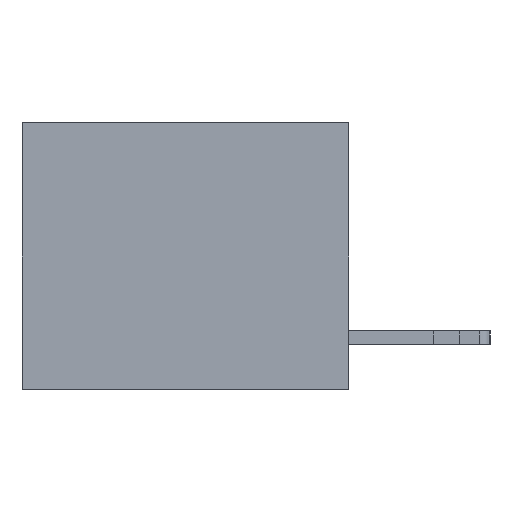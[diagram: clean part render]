
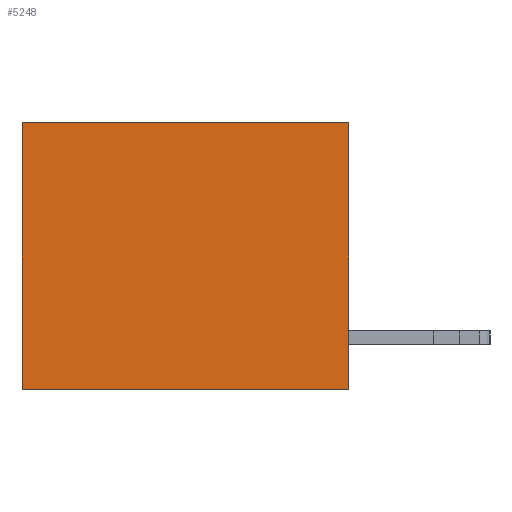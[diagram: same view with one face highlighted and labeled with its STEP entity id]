
A CAD part, left-side view. The second image highlights one B-rep face of the part: STEP entity #5248.
In plain terms, the highlighted planar face has unit normal (-1, 0, 0).
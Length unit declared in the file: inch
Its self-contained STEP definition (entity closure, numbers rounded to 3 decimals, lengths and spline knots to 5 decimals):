
#43 = CARTESIAN_POINT ( 'NONE',  ( 0.3165, 0., -0.49 ) ) ;
#988 = ORIENTED_EDGE ( 'NONE', *, *, #1631, .F. ) ;
#1576 = PLANE ( 'NONE',  #13339 ) ;
#1631 = EDGE_CURVE ( 'NONE', #11225, #2578, #13079, .T. ) ;
#2417 = LINE ( 'NONE', #6221, #11942 ) ;
#2578 = VERTEX_POINT ( 'NONE', #43 ) ;
#3488 = EDGE_LOOP ( 'NONE', ( #6164, #6166, #988, #10848 ) ) ;
#3574 = DIRECTION ( 'NONE',  ( 0., 0., -1. ) ) ;
#4277 = LINE ( 'NONE', #4351, #13620 ) ;
#4351 = CARTESIAN_POINT ( 'NONE',  ( 0.3165, 0., 0. ) ) ;
#4410 = EDGE_CURVE ( 'NONE', #2578, #6965, #11588, .T. ) ;
#5248 = ADVANCED_FACE ( 'NONE', ( #16947 ), #1576, .F. ) ;
#5443 = CARTESIAN_POINT ( 'NONE',  ( 0.3165, 0., -0.49 ) ) ;
#5701 = DIRECTION ( 'NONE',  ( 1., 0., 0. ) ) ;
#6164 = ORIENTED_EDGE ( 'NONE', *, *, #7230, .T. ) ;
#6166 = ORIENTED_EDGE ( 'NONE', *, *, #4410, .F. ) ;
#6221 = CARTESIAN_POINT ( 'NONE',  ( 0.3165, 0.6, -0.49 ) ) ;
#6637 = CARTESIAN_POINT ( 'NONE',  ( 0.3165, 0., -0.49 ) ) ;
#6726 = DIRECTION ( 'NONE',  ( 0., 1., 0. ) ) ;
#6937 = CARTESIAN_POINT ( 'NONE',  ( 0.3165, 0., -0.49 ) ) ;
#6965 = VERTEX_POINT ( 'NONE', #10193 ) ;
#7230 = EDGE_CURVE ( 'NONE', #10586, #6965, #2417, .T. ) ;
#7660 = VECTOR ( 'NONE', #6726, 39.37008 ) ;
#7778 = EDGE_CURVE ( 'NONE', #11225, #10586, #4277, .T. ) ;
#8551 = DIRECTION ( 'NONE',  ( 0., 1., 0. ) ) ;
#10102 = CARTESIAN_POINT ( 'NONE',  ( 0.3165, 0., 0. ) ) ;
#10193 = CARTESIAN_POINT ( 'NONE',  ( 0.3165, 0.6, -0.49 ) ) ;
#10586 = VERTEX_POINT ( 'NONE', #11004 ) ;
#10848 = ORIENTED_EDGE ( 'NONE', *, *, #7778, .T. ) ;
#10948 = DIRECTION ( 'NONE',  ( 0., 0., -1. ) ) ;
#11004 = CARTESIAN_POINT ( 'NONE',  ( 0.3165, 0.6, 0. ) ) ;
#11225 = VERTEX_POINT ( 'NONE', #10102 ) ;
#11588 = LINE ( 'NONE', #5443, #7660 ) ;
#11942 = VECTOR ( 'NONE', #3574, 39.37008 ) ;
#13079 = LINE ( 'NONE', #6637, #13696 ) ;
#13339 = AXIS2_PLACEMENT_3D ( 'NONE', #6937, #5701, #10948 ) ;
#13620 = VECTOR ( 'NONE', #8551, 39.37008 ) ;
#13696 = VECTOR ( 'NONE', #14390, 39.37008 ) ;
#14390 = DIRECTION ( 'NONE',  ( 0., 0., -1. ) ) ;
#16947 = FACE_OUTER_BOUND ( 'NONE', #3488, .T. ) ;
